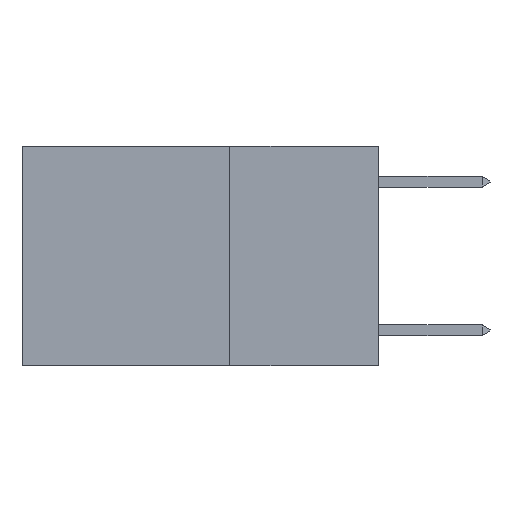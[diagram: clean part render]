
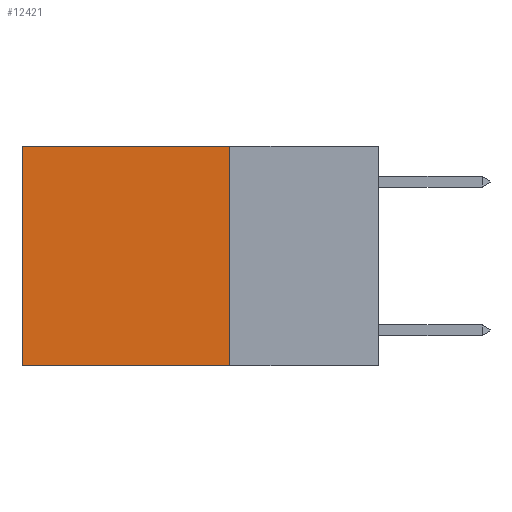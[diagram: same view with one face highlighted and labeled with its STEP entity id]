
A CAD part, left-side view. The second image highlights one B-rep face of the part: STEP entity #12421.
In plain terms, the highlighted planar face has unit normal (-1, 0, 0).
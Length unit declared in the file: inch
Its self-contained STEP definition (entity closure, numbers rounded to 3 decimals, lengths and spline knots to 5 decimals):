
#482 = CARTESIAN_POINT ( 'NONE',  ( 0.2625, 0.25, 0. ) ) ;
#741 = LINE ( 'NONE', #15509, #1574 ) ;
#1383 = DIRECTION ( 'NONE',  ( 1., 0., 0. ) ) ;
#1574 = VECTOR ( 'NONE', #2063, 39.37008 ) ;
#1844 = VERTEX_POINT ( 'NONE', #10690 ) ;
#2063 = DIRECTION ( 'NONE',  ( 0., 0., -1. ) ) ;
#3214 = EDGE_LOOP ( 'NONE', ( #21787, #8965, #15008, #20429 ) ) ;
#4048 = CARTESIAN_POINT ( 'NONE',  ( 0.2625, 0.25, 0. ) ) ;
#6156 = AXIS2_PLACEMENT_3D ( 'NONE', #4048, #1383, #12575 ) ;
#6314 = EDGE_CURVE ( 'NONE', #22789, #13918, #15422, .T. ) ;
#7434 = VECTOR ( 'NONE', #7977, 39.37008 ) ;
#7977 = DIRECTION ( 'NONE',  ( 0., 1., 0. ) ) ;
#8965 = ORIENTED_EDGE ( 'NONE', *, *, #13249, .F. ) ;
#10690 = CARTESIAN_POINT ( 'NONE',  ( 0.2625, 0.6, 0. ) ) ;
#12421 = ADVANCED_FACE ( 'NONE', ( #18376 ), #24313, .F. ) ;
#12575 = DIRECTION ( 'NONE',  ( 0., 0., -1. ) ) ;
#13073 = LINE ( 'NONE', #16563, #13641 ) ;
#13098 = VECTOR ( 'NONE', #15037, 39.37008 ) ;
#13157 = CARTESIAN_POINT ( 'NONE',  ( 0.2625, 0.6, -0.37 ) ) ;
#13249 = EDGE_CURVE ( 'NONE', #13918, #22401, #13073, .T. ) ;
#13634 = CARTESIAN_POINT ( 'NONE',  ( 0.2625, 0.25, 0. ) ) ;
#13641 = VECTOR ( 'NONE', #22124, 39.37008 ) ;
#13918 = VERTEX_POINT ( 'NONE', #15681 ) ;
#15008 = ORIENTED_EDGE ( 'NONE', *, *, #6314, .F. ) ;
#15037 = DIRECTION ( 'NONE',  ( 0., 0., -1. ) ) ;
#15422 = LINE ( 'NONE', #18963, #13098 ) ;
#15443 = EDGE_CURVE ( 'NONE', #22789, #1844, #17089, .T. ) ;
#15509 = CARTESIAN_POINT ( 'NONE',  ( 0.2625, 0.6, 0. ) ) ;
#15681 = CARTESIAN_POINT ( 'NONE',  ( 0.2625, 0.25, -0.37 ) ) ;
#16563 = CARTESIAN_POINT ( 'NONE',  ( 0.2625, 0.25, -0.37 ) ) ;
#16695 = EDGE_CURVE ( 'NONE', #1844, #22401, #741, .T. ) ;
#17089 = LINE ( 'NONE', #482, #7434 ) ;
#18376 = FACE_OUTER_BOUND ( 'NONE', #3214, .T. ) ;
#18963 = CARTESIAN_POINT ( 'NONE',  ( 0.2625, 0.25, 0. ) ) ;
#20429 = ORIENTED_EDGE ( 'NONE', *, *, #15443, .T. ) ;
#21787 = ORIENTED_EDGE ( 'NONE', *, *, #16695, .T. ) ;
#22124 = DIRECTION ( 'NONE',  ( 0., 1., 0. ) ) ;
#22401 = VERTEX_POINT ( 'NONE', #13157 ) ;
#22789 = VERTEX_POINT ( 'NONE', #13634 ) ;
#24313 = PLANE ( 'NONE',  #6156 ) ;
